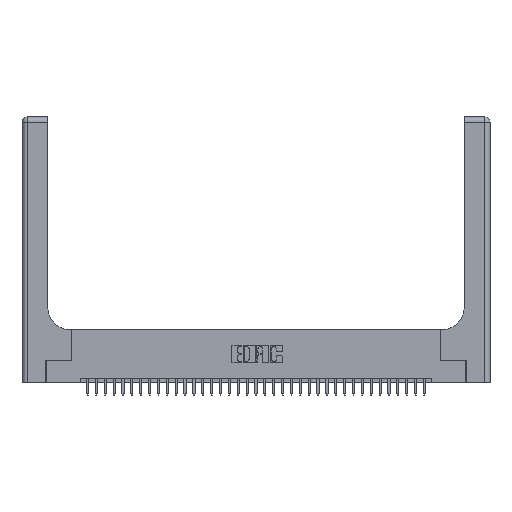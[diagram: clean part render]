
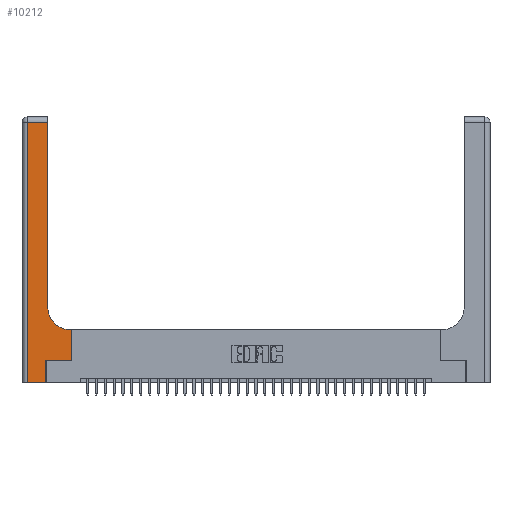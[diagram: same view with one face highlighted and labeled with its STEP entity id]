
A CAD part, top view. The second image highlights one B-rep face of the part: STEP entity #10212.
In plain terms, the highlighted planar face has unit normal (0, 0, 1).
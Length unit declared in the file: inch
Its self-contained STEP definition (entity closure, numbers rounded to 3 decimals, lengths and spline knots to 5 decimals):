
#375 = EDGE_CURVE ( 'NONE', #28485, #4401, #33451, .T. ) ;
#496 = CIRCLE ( 'NONE', #9375, 0.25 ) ;
#559 = LINE ( 'NONE', #26874, #29481 ) ;
#569 = CARTESIAN_POINT ( 'NONE',  ( 0.2915, 0.85, 0.37 ) ) ;
#741 = CARTESIAN_POINT ( 'NONE',  ( 0.2915, 3., 0.37 ) ) ;
#978 = DIRECTION ( 'NONE',  ( 0., 1., 0. ) ) ;
#1678 = VECTOR ( 'NONE', #7655, 39.37008 ) ;
#2267 = AXIS2_PLACEMENT_3D ( 'NONE', #10647, #2374, #32850 ) ;
#2374 = DIRECTION ( 'NONE',  ( 0., 0., -1. ) ) ;
#2875 = VERTEX_POINT ( 'NONE', #8830 ) ;
#3771 = ORIENTED_EDGE ( 'NONE', *, *, #8028, .T. ) ;
#4401 = VERTEX_POINT ( 'NONE', #11466 ) ;
#5143 = VECTOR ( 'NONE', #10701, 39.37008 ) ;
#5311 = VERTEX_POINT ( 'NONE', #11359 ) ;
#6395 = ORIENTED_EDGE ( 'NONE', *, *, #33249, .T. ) ;
#6834 = CARTESIAN_POINT ( 'NONE',  ( 0.5585, 0.25, 0.37 ) ) ;
#7362 = EDGE_CURVE ( 'NONE', #15395, #34570, #23045, .T. ) ;
#7655 = DIRECTION ( 'NONE',  ( -1., 0., 0. ) ) ;
#7688 = EDGE_CURVE ( 'NONE', #2875, #5311, #27452, .T. ) ;
#7985 = EDGE_CURVE ( 'NONE', #30860, #9901, #559, .T. ) ;
#8028 = EDGE_CURVE ( 'NONE', #5311, #28485, #496, .T. ) ;
#8830 = CARTESIAN_POINT ( 'NONE',  ( 0.5585, 0.6, 0.37 ) ) ;
#9184 = DIRECTION ( 'NONE',  ( -1., 0., 0. ) ) ;
#9375 = AXIS2_PLACEMENT_3D ( 'NONE', #29325, #11277, #30575 ) ;
#9901 = VERTEX_POINT ( 'NONE', #6834 ) ;
#10212 = ADVANCED_FACE ( 'NONE', ( #33471 ), #13208, .F. ) ;
#10647 = CARTESIAN_POINT ( 'NONE',  ( 0., 3., 0.37 ) ) ;
#10701 = DIRECTION ( 'NONE',  ( 0., -1., 0. ) ) ;
#11165 = CARTESIAN_POINT ( 'NONE',  ( 0.06, 2.94, 0.37 ) ) ;
#11277 = DIRECTION ( 'NONE',  ( 0., 0., -1. ) ) ;
#11359 = CARTESIAN_POINT ( 'NONE',  ( 0.5415, 0.6, 0.37 ) ) ;
#11466 = CARTESIAN_POINT ( 'NONE',  ( 0.2915, 2.94, 0.37 ) ) ;
#13208 = PLANE ( 'NONE',  #2267 ) ;
#13692 = VECTOR ( 'NONE', #978, 39.37008 ) ;
#13983 = EDGE_CURVE ( 'NONE', #9901, #2875, #21886, .T. ) ;
#14108 = CARTESIAN_POINT ( 'NONE',  ( 0.269, 0., 0.37 ) ) ;
#14262 = ORIENTED_EDGE ( 'NONE', *, *, #7688, .T. ) ;
#14436 = DIRECTION ( 'NONE',  ( 0., 1., 0. ) ) ;
#14673 = LINE ( 'NONE', #14108, #36225 ) ;
#14720 = ORIENTED_EDGE ( 'NONE', *, *, #7362, .T. ) ;
#15395 = VERTEX_POINT ( 'NONE', #11165 ) ;
#16266 = CARTESIAN_POINT ( 'NONE',  ( 0.2915, 0.6, 0.37 ) ) ;
#16837 = DIRECTION ( 'NONE',  ( 0., 1., 0. ) ) ;
#16966 = VERTEX_POINT ( 'NONE', #24453 ) ;
#17759 = VECTOR ( 'NONE', #9184, 39.37008 ) ;
#18312 = VECTOR ( 'NONE', #14436, 39.37008 ) ;
#19011 = LINE ( 'NONE', #23650, #25993 ) ;
#19167 = EDGE_CURVE ( 'NONE', #4401, #15395, #34057, .T. ) ;
#21886 = LINE ( 'NONE', #23628, #18312 ) ;
#23045 = LINE ( 'NONE', #35848, #5143 ) ;
#23628 = CARTESIAN_POINT ( 'NONE',  ( 0.5585, 0.25, 0.37 ) ) ;
#23650 = CARTESIAN_POINT ( 'NONE',  ( 0., 0., 0.37 ) ) ;
#24315 = EDGE_LOOP ( 'NONE', ( #30394, #34156, #14720, #34195, #6395, #29605, #28630, #14262, #3771 ) ) ;
#24453 = CARTESIAN_POINT ( 'NONE',  ( 0.269, 0., 0.37 ) ) ;
#25993 = VECTOR ( 'NONE', #35014, 39.37008 ) ;
#26874 = CARTESIAN_POINT ( 'NONE',  ( 0.269, 0.25, 0.37 ) ) ;
#26995 = DIRECTION ( 'NONE',  ( 1., 0., 0. ) ) ;
#27452 = LINE ( 'NONE', #16266, #17759 ) ;
#28485 = VERTEX_POINT ( 'NONE', #569 ) ;
#28630 = ORIENTED_EDGE ( 'NONE', *, *, #13983, .T. ) ;
#29325 = CARTESIAN_POINT ( 'NONE',  ( 0.5415, 0.85, 0.37 ) ) ;
#29481 = VECTOR ( 'NONE', #26995, 39.37008 ) ;
#29605 = ORIENTED_EDGE ( 'NONE', *, *, #7985, .T. ) ;
#30283 = CARTESIAN_POINT ( 'NONE',  ( 0.269, 0.25, 0.37 ) ) ;
#30394 = ORIENTED_EDGE ( 'NONE', *, *, #375, .T. ) ;
#30575 = DIRECTION ( 'NONE',  ( 1., 0., 0. ) ) ;
#30860 = VERTEX_POINT ( 'NONE', #30283 ) ;
#32850 = DIRECTION ( 'NONE',  ( -1., 0., 0. ) ) ;
#33249 = EDGE_CURVE ( 'NONE', #16966, #30860, #14673, .T. ) ;
#33451 = LINE ( 'NONE', #741, #13692 ) ;
#33471 = FACE_OUTER_BOUND ( 'NONE', #24315, .T. ) ;
#34057 = LINE ( 'NONE', #35853, #1678 ) ;
#34156 = ORIENTED_EDGE ( 'NONE', *, *, #19167, .T. ) ;
#34195 = ORIENTED_EDGE ( 'NONE', *, *, #35217, .T. ) ;
#34570 = VERTEX_POINT ( 'NONE', #35565 ) ;
#35014 = DIRECTION ( 'NONE',  ( 1., 0., 0. ) ) ;
#35217 = EDGE_CURVE ( 'NONE', #34570, #16966, #19011, .T. ) ;
#35565 = CARTESIAN_POINT ( 'NONE',  ( 0.06, 0., 0.37 ) ) ;
#35848 = CARTESIAN_POINT ( 'NONE',  ( 0.06, 3., 0.37 ) ) ;
#35853 = CARTESIAN_POINT ( 'NONE',  ( 0., 2.94, 0.37 ) ) ;
#36225 = VECTOR ( 'NONE', #16837, 39.37008 ) ;
